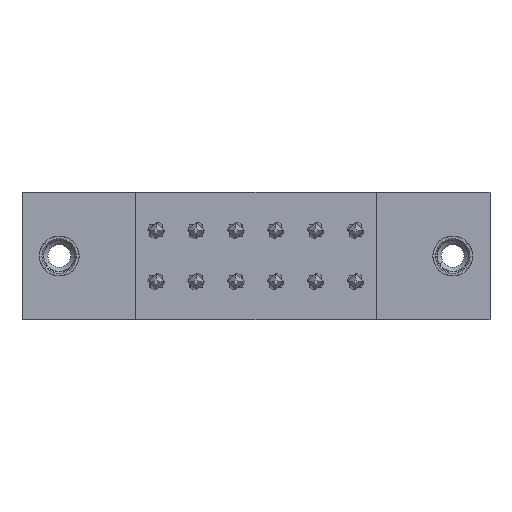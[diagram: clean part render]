
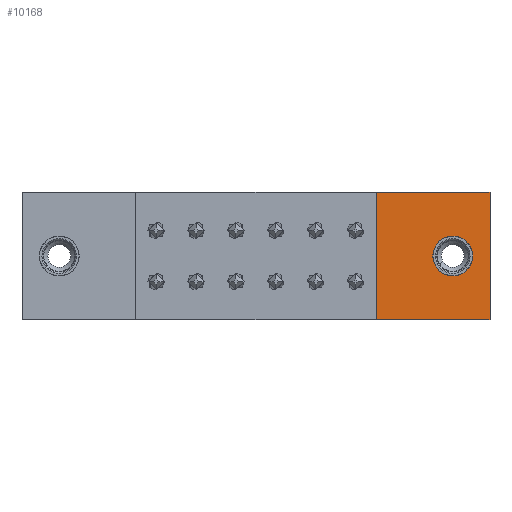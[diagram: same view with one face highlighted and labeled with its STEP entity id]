
A CAD part, front view. The second image highlights one B-rep face of the part: STEP entity #10168.
In plain terms, the highlighted planar face has unit normal (0, -1, 0).
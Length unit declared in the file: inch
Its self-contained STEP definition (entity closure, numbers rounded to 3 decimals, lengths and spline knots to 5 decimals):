
#406 = VERTEX_POINT ( 'NONE', #12824 ) ;
#592 = PLANE ( 'NONE',  #11890 ) ;
#802 = VERTEX_POINT ( 'NONE', #14593 ) ;
#1222 = CARTESIAN_POINT ( 'NONE',  ( 1.6845, 0.163, -0.25 ) ) ;
#1233 = CARTESIAN_POINT ( 'NONE',  ( 1.83, 0.163, -0.5 ) ) ;
#1562 = CARTESIAN_POINT ( 'NONE',  ( 1.385, 0.163, -0.5 ) ) ;
#2031 = VECTOR ( 'NONE', #4682, 39.37008 ) ;
#2324 = VECTOR ( 'NONE', #10224, 39.37008 ) ;
#2610 = VERTEX_POINT ( 'NONE', #9273 ) ;
#2668 = EDGE_LOOP ( 'NONE', ( #2925, #14630, #3475, #4868 ) ) ;
#2716 = VECTOR ( 'NONE', #12623, 39.37008 ) ;
#2791 = CARTESIAN_POINT ( 'NONE',  ( 1.6845, 0.163, -0.25 ) ) ;
#2925 = ORIENTED_EDGE ( 'NONE', *, *, #8559, .T. ) ;
#3000 = CARTESIAN_POINT ( 'NONE',  ( 1.83, 0.163, 0. ) ) ;
#3062 = CARTESIAN_POINT ( 'NONE',  ( 1.385, 0.163, -0.5 ) ) ;
#3240 = CIRCLE ( 'NONE', #9330, 0.078 ) ;
#3430 = DIRECTION ( 'NONE',  ( 0., 1., 0. ) ) ;
#3475 = ORIENTED_EDGE ( 'NONE', *, *, #9739, .T. ) ;
#4500 = VECTOR ( 'NONE', #6494, 39.37008 ) ;
#4526 = VERTEX_POINT ( 'NONE', #1562 ) ;
#4616 = CARTESIAN_POINT ( 'NONE',  ( 1.83, 0.163, 0. ) ) ;
#4682 = DIRECTION ( 'NONE',  ( 0., 0., 1. ) ) ;
#4868 = ORIENTED_EDGE ( 'NONE', *, *, #12116, .T. ) ;
#4921 = AXIS2_PLACEMENT_3D ( 'NONE', #2791, #7293, #11722 ) ;
#6458 = EDGE_CURVE ( 'NONE', #8444, #2610, #11968, .T. ) ;
#6494 = DIRECTION ( 'NONE',  ( 0., 0., -1. ) ) ;
#6531 = DIRECTION ( 'NONE',  ( 0., -1., 0. ) ) ;
#6680 = FACE_BOUND ( 'NONE', #11515, .T. ) ;
#7293 = DIRECTION ( 'NONE',  ( 0., 1., 0. ) ) ;
#7373 = ORIENTED_EDGE ( 'NONE', *, *, #10395, .T. ) ;
#7494 = DIRECTION ( 'NONE',  ( 0., 0., -1. ) ) ;
#8188 = LINE ( 'NONE', #1233, #2031 ) ;
#8444 = VERTEX_POINT ( 'NONE', #12083 ) ;
#8559 = EDGE_CURVE ( 'NONE', #802, #13875, #8188, .T. ) ;
#9087 = ORIENTED_EDGE ( 'NONE', *, *, #6458, .T. ) ;
#9251 = DIRECTION ( 'NONE',  ( 0., 0., -1. ) ) ;
#9273 = CARTESIAN_POINT ( 'NONE',  ( 1.6845, 0.163, -0.172 ) ) ;
#9330 = AXIS2_PLACEMENT_3D ( 'NONE', #1222, #3430, #9251 ) ;
#9739 = EDGE_CURVE ( 'NONE', #406, #4526, #12244, .T. ) ;
#10168 = ADVANCED_FACE ( 'NONE', ( #13322, #6680 ), #592, .T. ) ;
#10224 = DIRECTION ( 'NONE',  ( 1., 0., 0. ) ) ;
#10358 = EDGE_CURVE ( 'NONE', #13875, #406, #10814, .T. ) ;
#10395 = EDGE_CURVE ( 'NONE', #2610, #8444, #3240, .T. ) ;
#10814 = LINE ( 'NONE', #4616, #2716 ) ;
#11515 = EDGE_LOOP ( 'NONE', ( #7373, #9087 ) ) ;
#11722 = DIRECTION ( 'NONE',  ( 0., 0., -1. ) ) ;
#11890 = AXIS2_PLACEMENT_3D ( 'NONE', #3000, #6531, #7494 ) ;
#11968 = CIRCLE ( 'NONE', #4921, 0.078 ) ;
#12083 = CARTESIAN_POINT ( 'NONE',  ( 1.6845, 0.163, -0.328 ) ) ;
#12116 = EDGE_CURVE ( 'NONE', #4526, #802, #14182, .T. ) ;
#12244 = LINE ( 'NONE', #3062, #4500 ) ;
#12623 = DIRECTION ( 'NONE',  ( -1., 0., 0. ) ) ;
#12726 = CARTESIAN_POINT ( 'NONE',  ( 1.83, 0.163, 0. ) ) ;
#12824 = CARTESIAN_POINT ( 'NONE',  ( 1.385, 0.163, 0. ) ) ;
#13322 = FACE_OUTER_BOUND ( 'NONE', #2668, .T. ) ;
#13875 = VERTEX_POINT ( 'NONE', #12726 ) ;
#14182 = LINE ( 'NONE', #14313, #2324 ) ;
#14313 = CARTESIAN_POINT ( 'NONE',  ( 1.83, 0.163, -0.5 ) ) ;
#14593 = CARTESIAN_POINT ( 'NONE',  ( 1.83, 0.163, -0.5 ) ) ;
#14630 = ORIENTED_EDGE ( 'NONE', *, *, #10358, .T. ) ;
